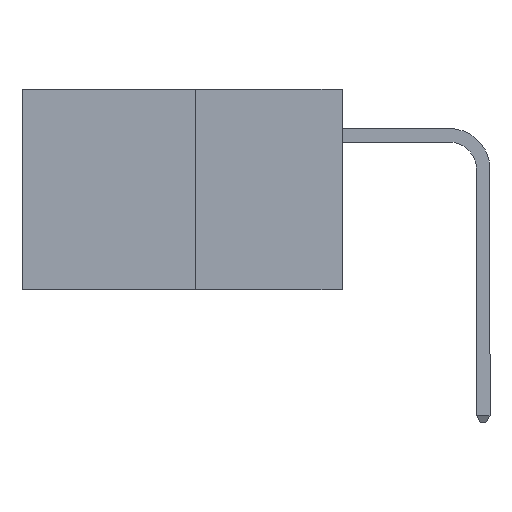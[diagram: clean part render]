
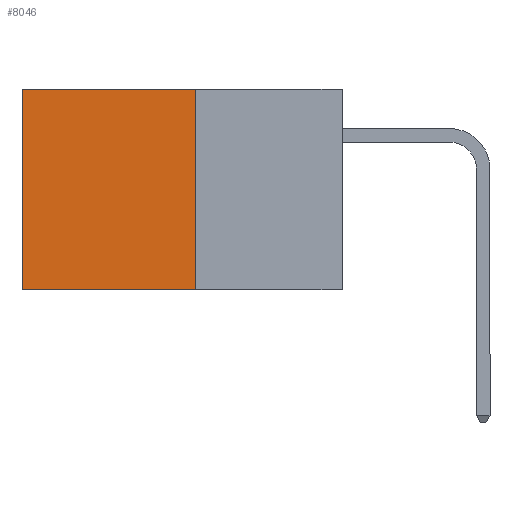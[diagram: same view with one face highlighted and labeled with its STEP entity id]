
A CAD part, left-side view. The second image highlights one B-rep face of the part: STEP entity #8046.
In plain terms, the highlighted planar face has unit normal (-1, 0, 0).
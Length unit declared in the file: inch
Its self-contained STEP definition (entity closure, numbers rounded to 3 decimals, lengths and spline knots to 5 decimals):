
#358 = LINE ( 'NONE', #27879, #29677 ) ;
#673 = DIRECTION ( 'NONE',  ( 0., 1., 0. ) ) ;
#1115 = AXIS2_PLACEMENT_3D ( 'NONE', #18215, #20488, #6553 ) ;
#1156 = ORIENTED_EDGE ( 'NONE', *, *, #20170, .T. ) ;
#1371 = VERTEX_POINT ( 'NONE', #19164 ) ;
#1667 = PLANE ( 'NONE',  #1115 ) ;
#2689 = ORIENTED_EDGE ( 'NONE', *, *, #26869, .F. ) ;
#3622 = FACE_OUTER_BOUND ( 'NONE', #26562, .T. ) ;
#4936 = DIRECTION ( 'NONE',  ( 0., 1., 0. ) ) ;
#5116 = EDGE_CURVE ( 'NONE', #5242, #24230, #18906, .T. ) ;
#5242 = VERTEX_POINT ( 'NONE', #10907 ) ;
#5383 = VECTOR ( 'NONE', #17141, 39.37008 ) ;
#6323 = ORIENTED_EDGE ( 'NONE', *, *, #13372, .T. ) ;
#6553 = DIRECTION ( 'NONE',  ( 0., 0., -1. ) ) ;
#8046 = ADVANCED_FACE ( 'NONE', ( #3622 ), #1667, .F. ) ;
#10063 = DIRECTION ( 'NONE',  ( 0., 0., -1. ) ) ;
#10461 = CARTESIAN_POINT ( 'NONE',  ( 0.277, 0.27, -0.37 ) ) ;
#10907 = CARTESIAN_POINT ( 'NONE',  ( 0.277, 0.27, 0. ) ) ;
#12077 = VECTOR ( 'NONE', #673, 39.37008 ) ;
#12529 = CARTESIAN_POINT ( 'NONE',  ( 0.277, 0.59, -0.37 ) ) ;
#12805 = VECTOR ( 'NONE', #10063, 39.37008 ) ;
#13372 = EDGE_CURVE ( 'NONE', #5242, #1371, #358, .T. ) ;
#14482 = VERTEX_POINT ( 'NONE', #15226 ) ;
#15226 = CARTESIAN_POINT ( 'NONE',  ( 0.277, 0.59, -0.37 ) ) ;
#16473 = CARTESIAN_POINT ( 'NONE',  ( 0.277, 0.27, -0.37 ) ) ;
#17141 = DIRECTION ( 'NONE',  ( 0., 0., -1. ) ) ;
#17888 = LINE ( 'NONE', #12529, #5383 ) ;
#18215 = CARTESIAN_POINT ( 'NONE',  ( 0.277, 0.27, -0.37 ) ) ;
#18906 = LINE ( 'NONE', #16473, #12805 ) ;
#19164 = CARTESIAN_POINT ( 'NONE',  ( 0.277, 0.59, 0. ) ) ;
#19590 = LINE ( 'NONE', #28461, #12077 ) ;
#20170 = EDGE_CURVE ( 'NONE', #1371, #14482, #17888, .T. ) ;
#20488 = DIRECTION ( 'NONE',  ( 1., 0., 0. ) ) ;
#24230 = VERTEX_POINT ( 'NONE', #10461 ) ;
#25433 = ORIENTED_EDGE ( 'NONE', *, *, #5116, .F. ) ;
#26562 = EDGE_LOOP ( 'NONE', ( #1156, #2689, #25433, #6323 ) ) ;
#26869 = EDGE_CURVE ( 'NONE', #24230, #14482, #19590, .T. ) ;
#27879 = CARTESIAN_POINT ( 'NONE',  ( 0.277, 0.27, 0. ) ) ;
#28461 = CARTESIAN_POINT ( 'NONE',  ( 0.277, 0.27, -0.37 ) ) ;
#29677 = VECTOR ( 'NONE', #4936, 39.37008 ) ;
